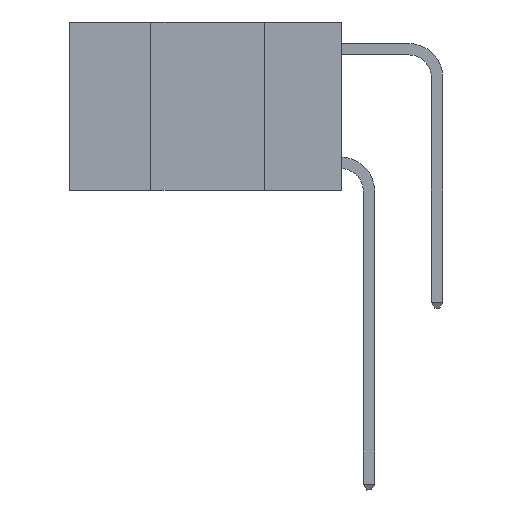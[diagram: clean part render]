
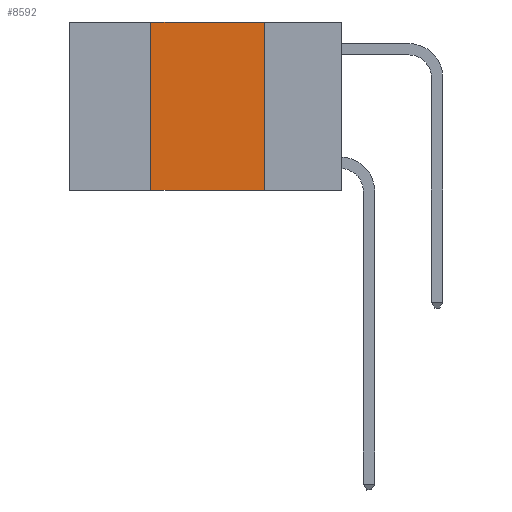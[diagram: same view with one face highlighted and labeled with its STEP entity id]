
A CAD part, left-side view. The second image highlights one B-rep face of the part: STEP entity #8592.
In plain terms, the highlighted planar face has unit normal (-1, 0, 0).
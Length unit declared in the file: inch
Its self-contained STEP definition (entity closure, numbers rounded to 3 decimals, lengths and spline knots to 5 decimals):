
#416 = VERTEX_POINT ( 'NONE', #10670 ) ;
#1394 = LINE ( 'NONE', #9579, #9470 ) ;
#2109 = VERTEX_POINT ( 'NONE', #12061 ) ;
#2404 = CARTESIAN_POINT ( 'NONE',  ( 0., 0.6, 0. ) ) ;
#2691 = DIRECTION ( 'NONE',  ( 0., -1., 0. ) ) ;
#3717 = FACE_OUTER_BOUND ( 'NONE', #11932, .T. ) ;
#4527 = ORIENTED_EDGE ( 'NONE', *, *, #7507, .F. ) ;
#4540 = VERTEX_POINT ( 'NONE', #7172 ) ;
#4747 = VECTOR ( 'NONE', #4995, 39.37008 ) ;
#4995 = DIRECTION ( 'NONE',  ( 0., 0., -1. ) ) ;
#5275 = ORIENTED_EDGE ( 'NONE', *, *, #14351, .F. ) ;
#5758 = AXIS2_PLACEMENT_3D ( 'NONE', #2404, #11442, #13747 ) ;
#5917 = VECTOR ( 'NONE', #14722, 39.37008 ) ;
#7172 = CARTESIAN_POINT ( 'NONE',  ( 0., 0.42, 0. ) ) ;
#7359 = EDGE_CURVE ( 'NONE', #10813, #2109, #1394, .T. ) ;
#7507 = EDGE_CURVE ( 'NONE', #4540, #416, #12857, .T. ) ;
#7555 = EDGE_CURVE ( 'NONE', #10813, #4540, #13931, .T. ) ;
#7584 = CARTESIAN_POINT ( 'NONE',  ( 0., 0.6, 0. ) ) ;
#8246 = PLANE ( 'NONE',  #5758 ) ;
#8592 = ADVANCED_FACE ( 'NONE', ( #3717 ), #8246, .F. ) ;
#8723 = DIRECTION ( 'NONE',  ( 0., -1., 0. ) ) ;
#8819 = ORIENTED_EDGE ( 'NONE', *, *, #7555, .F. ) ;
#9277 = ORIENTED_EDGE ( 'NONE', *, *, #7359, .T. ) ;
#9470 = VECTOR ( 'NONE', #2691, 39.37008 ) ;
#9579 = CARTESIAN_POINT ( 'NONE',  ( 0., 0.6, -0.37 ) ) ;
#10645 = CARTESIAN_POINT ( 'NONE',  ( 0., 0.42, -0.37 ) ) ;
#10670 = CARTESIAN_POINT ( 'NONE',  ( 0., 0.17, 0. ) ) ;
#10813 = VERTEX_POINT ( 'NONE', #10645 ) ;
#11442 = DIRECTION ( 'NONE',  ( 1., 0., 0. ) ) ;
#11803 = CARTESIAN_POINT ( 'NONE',  ( 0., 0.17, 0. ) ) ;
#11932 = EDGE_LOOP ( 'NONE', ( #5275, #4527, #8819, #9277 ) ) ;
#11955 = VECTOR ( 'NONE', #8723, 39.37008 ) ;
#12061 = CARTESIAN_POINT ( 'NONE',  ( 0., 0.17, -0.37 ) ) ;
#12857 = LINE ( 'NONE', #7584, #11955 ) ;
#13639 = CARTESIAN_POINT ( 'NONE',  ( 0., 0.42, 0. ) ) ;
#13747 = DIRECTION ( 'NONE',  ( 0., 0., -1. ) ) ;
#13931 = LINE ( 'NONE', #13639, #5917 ) ;
#14009 = LINE ( 'NONE', #11803, #4747 ) ;
#14351 = EDGE_CURVE ( 'NONE', #416, #2109, #14009, .T. ) ;
#14722 = DIRECTION ( 'NONE',  ( 0., 0., 1. ) ) ;
